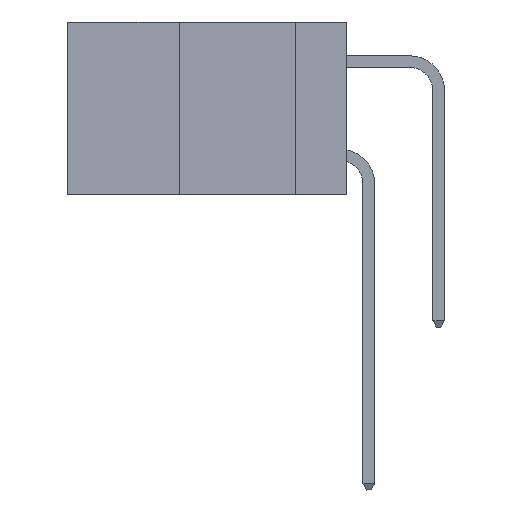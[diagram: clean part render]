
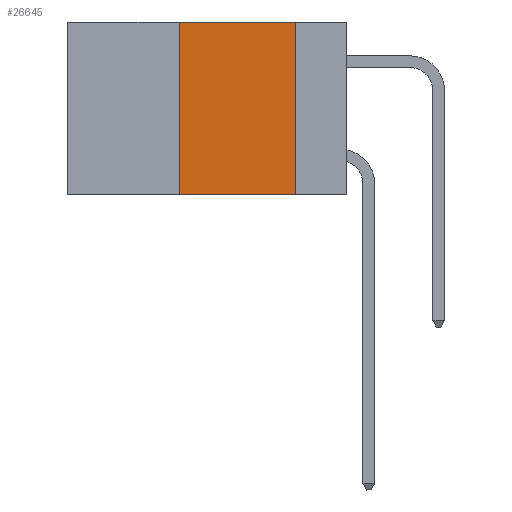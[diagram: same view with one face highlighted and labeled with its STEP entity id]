
A CAD part, left-side view. The second image highlights one B-rep face of the part: STEP entity #26645.
In plain terms, the highlighted planar face has unit normal (-1, 0, 0).
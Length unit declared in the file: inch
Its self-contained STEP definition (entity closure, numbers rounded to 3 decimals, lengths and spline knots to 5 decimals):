
#618 = VECTOR ( 'NONE', #26598, 39.37008 ) ;
#2827 = DIRECTION ( 'NONE',  ( 1., 0., 0. ) ) ;
#2961 = VERTEX_POINT ( 'NONE', #18784 ) ;
#3377 = VERTEX_POINT ( 'NONE', #20785 ) ;
#4012 = CARTESIAN_POINT ( 'NONE',  ( 0., 0.36, 0. ) ) ;
#4662 = EDGE_LOOP ( 'NONE', ( #9853, #21942, #16849, #27724 ) ) ;
#4877 = VECTOR ( 'NONE', #17907, 39.37008 ) ;
#5682 = LINE ( 'NONE', #4012, #16493 ) ;
#6129 = VECTOR ( 'NONE', #21318, 39.37008 ) ;
#9161 = EDGE_CURVE ( 'NONE', #3377, #9966, #11888, .T. ) ;
#9853 = ORIENTED_EDGE ( 'NONE', *, *, #10141, .F. ) ;
#9966 = VERTEX_POINT ( 'NONE', #28340 ) ;
#10141 = EDGE_CURVE ( 'NONE', #14715, #9966, #13828, .T. ) ;
#11768 = EDGE_CURVE ( 'NONE', #3377, #2961, #5682, .T. ) ;
#11888 = LINE ( 'NONE', #22780, #4877 ) ;
#13828 = LINE ( 'NONE', #19080, #6129 ) ;
#14715 = VERTEX_POINT ( 'NONE', #21740 ) ;
#14787 = EDGE_CURVE ( 'NONE', #2961, #14715, #26328, .T. ) ;
#15141 = AXIS2_PLACEMENT_3D ( 'NONE', #16238, #2827, #18498 ) ;
#16238 = CARTESIAN_POINT ( 'NONE',  ( 0., 0.6, 0. ) ) ;
#16493 = VECTOR ( 'NONE', #23933, 39.37008 ) ;
#16849 = ORIENTED_EDGE ( 'NONE', *, *, #11768, .F. ) ;
#17076 = CARTESIAN_POINT ( 'NONE',  ( 0., 0.6, 0. ) ) ;
#17907 = DIRECTION ( 'NONE',  ( 0., -1., 0. ) ) ;
#18498 = DIRECTION ( 'NONE',  ( 0., 0., -1. ) ) ;
#18784 = CARTESIAN_POINT ( 'NONE',  ( 0., 0.36, 0. ) ) ;
#19080 = CARTESIAN_POINT ( 'NONE',  ( 0., 0.11, 0. ) ) ;
#20785 = CARTESIAN_POINT ( 'NONE',  ( 0., 0.36, -0.37 ) ) ;
#21318 = DIRECTION ( 'NONE',  ( 0., 0., -1. ) ) ;
#21740 = CARTESIAN_POINT ( 'NONE',  ( 0., 0.11, 0. ) ) ;
#21815 = FACE_OUTER_BOUND ( 'NONE', #4662, .T. ) ;
#21942 = ORIENTED_EDGE ( 'NONE', *, *, #14787, .F. ) ;
#22780 = CARTESIAN_POINT ( 'NONE',  ( 0., 0.6, -0.37 ) ) ;
#23933 = DIRECTION ( 'NONE',  ( 0., 0., 1. ) ) ;
#25100 = PLANE ( 'NONE',  #15141 ) ;
#26328 = LINE ( 'NONE', #17076, #618 ) ;
#26598 = DIRECTION ( 'NONE',  ( 0., -1., 0. ) ) ;
#26645 = ADVANCED_FACE ( 'NONE', ( #21815 ), #25100, .F. ) ;
#27724 = ORIENTED_EDGE ( 'NONE', *, *, #9161, .T. ) ;
#28340 = CARTESIAN_POINT ( 'NONE',  ( 0., 0.11, -0.37 ) ) ;
